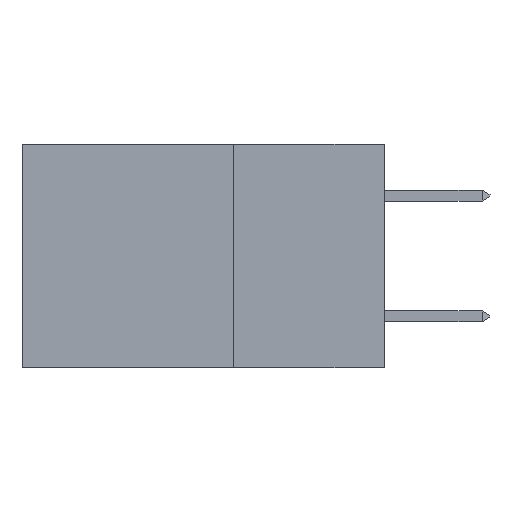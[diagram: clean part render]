
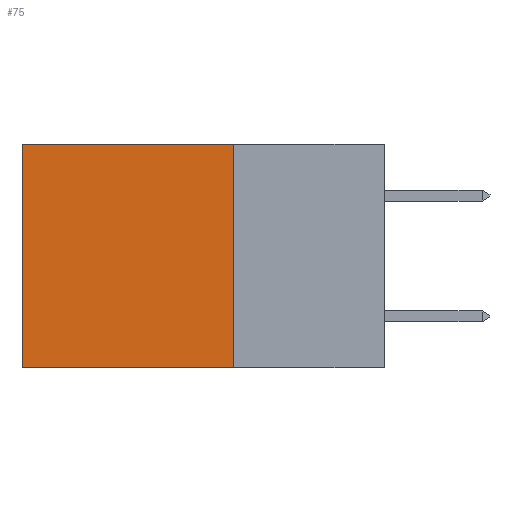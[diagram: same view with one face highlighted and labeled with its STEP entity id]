
A CAD part, left-side view. The second image highlights one B-rep face of the part: STEP entity #75.
In plain terms, the highlighted planar face has unit normal (-1, 0, 0).
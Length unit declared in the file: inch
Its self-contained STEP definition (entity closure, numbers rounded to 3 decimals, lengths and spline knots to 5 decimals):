
#48 = EDGE_CURVE ( 'NONE', #2440, #1278, #3485, .T. ) ;
#75 = ADVANCED_FACE ( 'NONE', ( #12535 ), #6092, .F. ) ;
#455 = DIRECTION ( 'NONE',  ( 0., 0., -1. ) ) ;
#576 = CARTESIAN_POINT ( 'NONE',  ( 0.2875, 0.25, 0. ) ) ;
#851 = DIRECTION ( 'NONE',  ( 1., 0., 0. ) ) ;
#1163 = CARTESIAN_POINT ( 'NONE',  ( 0.2875, 0.25, -0.37 ) ) ;
#1278 = VERTEX_POINT ( 'NONE', #3899 ) ;
#1449 = VECTOR ( 'NONE', #1914, 39.37008 ) ;
#1474 = VERTEX_POINT ( 'NONE', #7278 ) ;
#1793 = ORIENTED_EDGE ( 'NONE', *, *, #11361, .T. ) ;
#1914 = DIRECTION ( 'NONE',  ( 0., 0., -1. ) ) ;
#2149 = ORIENTED_EDGE ( 'NONE', *, *, #48, .F. ) ;
#2167 = ORIENTED_EDGE ( 'NONE', *, *, #10914, .F. ) ;
#2440 = VERTEX_POINT ( 'NONE', #9682 ) ;
#2636 = LINE ( 'NONE', #576, #9102 ) ;
#3336 = EDGE_LOOP ( 'NONE', ( #1793, #2149, #2167, #4161 ) ) ;
#3485 = LINE ( 'NONE', #1163, #6693 ) ;
#3899 = CARTESIAN_POINT ( 'NONE',  ( 0.2875, 0.6, -0.37 ) ) ;
#4161 = ORIENTED_EDGE ( 'NONE', *, *, #7659, .T. ) ;
#5873 = DIRECTION ( 'NONE',  ( 0., 0., -1. ) ) ;
#5977 = VECTOR ( 'NONE', #5873, 39.37008 ) ;
#6092 = PLANE ( 'NONE',  #13198 ) ;
#6693 = VECTOR ( 'NONE', #7287, 39.37008 ) ;
#7149 = CARTESIAN_POINT ( 'NONE',  ( 0.2875, 0.25, 0. ) ) ;
#7278 = CARTESIAN_POINT ( 'NONE',  ( 0.2875, 0.25, 0. ) ) ;
#7287 = DIRECTION ( 'NONE',  ( 0., 1., 0. ) ) ;
#7659 = EDGE_CURVE ( 'NONE', #1474, #13068, #2636, .T. ) ;
#7688 = CARTESIAN_POINT ( 'NONE',  ( 0.2875, 0.25, 0. ) ) ;
#8296 = CARTESIAN_POINT ( 'NONE',  ( 0.2875, 0.6, 0. ) ) ;
#9102 = VECTOR ( 'NONE', #9246, 39.37008 ) ;
#9246 = DIRECTION ( 'NONE',  ( 0., 1., 0. ) ) ;
#9682 = CARTESIAN_POINT ( 'NONE',  ( 0.2875, 0.25, -0.37 ) ) ;
#10423 = CARTESIAN_POINT ( 'NONE',  ( 0.2875, 0.6, 0. ) ) ;
#10465 = LINE ( 'NONE', #10423, #1449 ) ;
#10842 = LINE ( 'NONE', #7149, #5977 ) ;
#10914 = EDGE_CURVE ( 'NONE', #1474, #2440, #10842, .T. ) ;
#11361 = EDGE_CURVE ( 'NONE', #13068, #1278, #10465, .T. ) ;
#12535 = FACE_OUTER_BOUND ( 'NONE', #3336, .T. ) ;
#13068 = VERTEX_POINT ( 'NONE', #8296 ) ;
#13198 = AXIS2_PLACEMENT_3D ( 'NONE', #7688, #851, #455 ) ;
